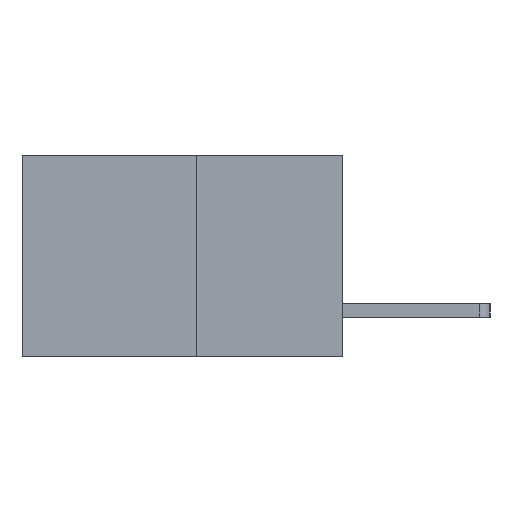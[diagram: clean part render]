
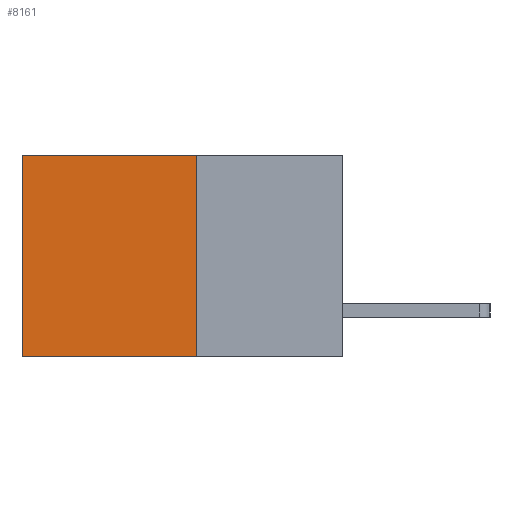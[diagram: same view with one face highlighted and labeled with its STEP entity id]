
A CAD part, left-side view. The second image highlights one B-rep face of the part: STEP entity #8161.
In plain terms, the highlighted planar face has unit normal (-1, 0, 0).
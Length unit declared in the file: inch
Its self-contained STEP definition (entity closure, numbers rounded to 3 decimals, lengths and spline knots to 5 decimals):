
#185 = VERTEX_POINT ( 'NONE', #6108 ) ;
#220 = PLANE ( 'NONE',  #11055 ) ;
#553 = FACE_OUTER_BOUND ( 'NONE', #4642, .T. ) ;
#1034 = ORIENTED_EDGE ( 'NONE', *, *, #8927, .T. ) ;
#1041 = VECTOR ( 'NONE', #7126, 39.37008 ) ;
#1049 = ORIENTED_EDGE ( 'NONE', *, *, #9770, .F. ) ;
#1082 = ORIENTED_EDGE ( 'NONE', *, *, #6769, .F. ) ;
#1113 = ORIENTED_EDGE ( 'NONE', *, *, #4738, .T. ) ;
#1263 = CARTESIAN_POINT ( 'NONE',  ( 0.277, 0.27, -0.37 ) ) ;
#1305 = DIRECTION ( 'NONE',  ( 0., 0., -1. ) ) ;
#1725 = CARTESIAN_POINT ( 'NONE',  ( 0.277, 0.59, -0.37 ) ) ;
#2389 = LINE ( 'NONE', #3142, #12776 ) ;
#2495 = CARTESIAN_POINT ( 'NONE',  ( 0.277, 0.27, -0.37 ) ) ;
#3142 = CARTESIAN_POINT ( 'NONE',  ( 0.277, 0.27, -0.37 ) ) ;
#4248 = DIRECTION ( 'NONE',  ( 0., 0., -1. ) ) ;
#4479 = CARTESIAN_POINT ( 'NONE',  ( 0.277, 0.27, -0.37 ) ) ;
#4642 = EDGE_LOOP ( 'NONE', ( #1034, #1049, #1082, #1113 ) ) ;
#4738 = EDGE_CURVE ( 'NONE', #12895, #185, #11315, .T. ) ;
#4740 = LINE ( 'NONE', #4479, #9782 ) ;
#4763 = VECTOR ( 'NONE', #9003, 39.37008 ) ;
#5260 = DIRECTION ( 'NONE',  ( 0., 1., 0. ) ) ;
#6108 = CARTESIAN_POINT ( 'NONE',  ( 0.277, 0.59, 0. ) ) ;
#6550 = CARTESIAN_POINT ( 'NONE',  ( 0.277, 0.27, 0. ) ) ;
#6769 = EDGE_CURVE ( 'NONE', #12895, #8208, #4740, .T. ) ;
#7123 = CARTESIAN_POINT ( 'NONE',  ( 0.277, 0.27, 0. ) ) ;
#7126 = DIRECTION ( 'NONE',  ( 0., 1., 0. ) ) ;
#7630 = DIRECTION ( 'NONE',  ( 1., 0., 0. ) ) ;
#7814 = LINE ( 'NONE', #1725, #4763 ) ;
#8161 = ADVANCED_FACE ( 'NONE', ( #553 ), #220, .F. ) ;
#8208 = VERTEX_POINT ( 'NONE', #2495 ) ;
#8927 = EDGE_CURVE ( 'NONE', #185, #10475, #7814, .T. ) ;
#9003 = DIRECTION ( 'NONE',  ( 0., 0., -1. ) ) ;
#9770 = EDGE_CURVE ( 'NONE', #8208, #10475, #2389, .T. ) ;
#9782 = VECTOR ( 'NONE', #4248, 39.37008 ) ;
#10475 = VERTEX_POINT ( 'NONE', #11596 ) ;
#11055 = AXIS2_PLACEMENT_3D ( 'NONE', #1263, #7630, #1305 ) ;
#11315 = LINE ( 'NONE', #7123, #1041 ) ;
#11596 = CARTESIAN_POINT ( 'NONE',  ( 0.277, 0.59, -0.37 ) ) ;
#12776 = VECTOR ( 'NONE', #5260, 39.37008 ) ;
#12895 = VERTEX_POINT ( 'NONE', #6550 ) ;
